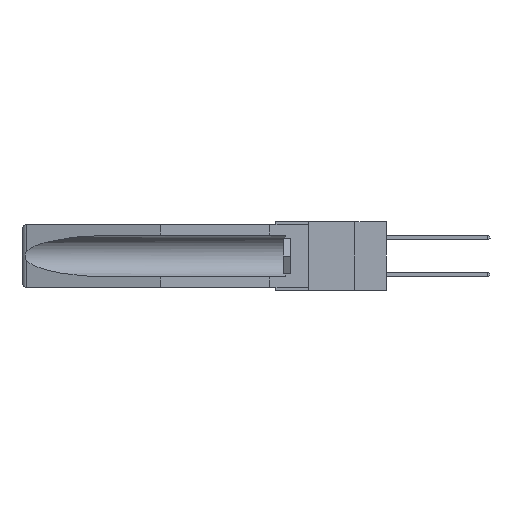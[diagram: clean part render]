
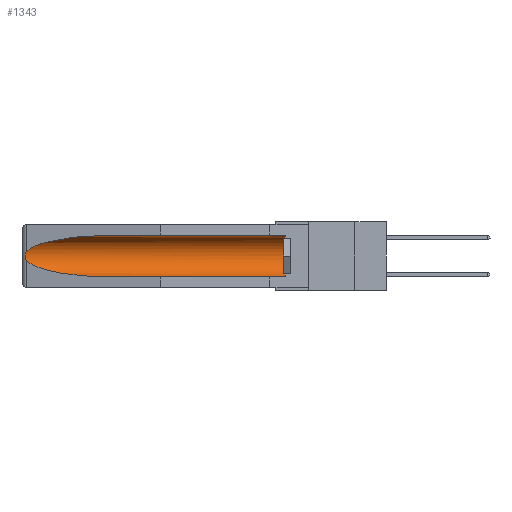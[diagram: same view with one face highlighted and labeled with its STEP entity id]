
A CAD part, left-side view. The second image highlights one B-rep face of the part: STEP entity #1343.
In plain terms, the highlighted cylindrical face has radius 2.857 mm (diameter 5.715 mm), a partial arc.
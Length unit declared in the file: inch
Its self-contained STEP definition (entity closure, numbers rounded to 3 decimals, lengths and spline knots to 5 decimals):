
#374 = CARTESIAN_POINT ( 'NONE',  ( 0.155, -0.30754, -0.284 ) ) ;
#415 = VECTOR ( 'NONE', #24213, 39.37008 ) ;
#1343 = ADVANCED_FACE ( 'NONE', ( #32321 ), #10674, .F. ) ;
#1872 = CARTESIAN_POINT ( 'NONE',  ( 0.155, 0.126, -0.284 ) ) ;
#2726 = EDGE_CURVE ( 'NONE', #32464, #9034, #24548, .T. ) ;
#3020 = CARTESIAN_POINT ( 'NONE',  ( 0.155, -0.30754, -0.1715 ) ) ;
#3129 = DIRECTION ( 'NONE',  ( 0., 1., 0. ) ) ;
#5174 = EDGE_CURVE ( 'NONE', #14724, #9034, #23425, .T. ) ;
#5193 = CARTESIAN_POINT ( 'NONE',  ( 0.155, 1.07973, -0.059 ) ) ;
#5306 = CARTESIAN_POINT ( 'NONE',  ( 0.155, 1.07973, -0.284 ) ) ;
#6300 = VECTOR ( 'NONE', #32778, 39.37008 ) ;
#6371 = DIRECTION ( 'NONE',  ( 0., 0., 1. ) ) ;
#7071 = CARTESIAN_POINT ( 'NONE',  ( 0.155, 0.126, -0.059 ) ) ;
#7737 = CARTESIAN_POINT ( 'NONE',  ( 0.26537, 1.52718, -0.14972 ) ) ;
#7749 = CARTESIAN_POINT ( 'NONE',  ( 0.26537, 1.52718, -0.19328 ) ) ;
#8071 = CARTESIAN_POINT ( 'NONE',  ( 0.26537, 1.52718, -0.19328 ) ) ;
#8982 = VERTEX_POINT ( 'NONE', #10057 ) ;
#9034 = VERTEX_POINT ( 'NONE', #15306 ) ;
#9903 = CARTESIAN_POINT ( 'NONE',  ( 0.26537, 1.52718, -0.14972 ) ) ;
#9992 = EDGE_CURVE ( 'NONE', #14724, #17891, #33779, .T. ) ;
#10057 = CARTESIAN_POINT ( 'NONE',  ( 0.155, 1.07973, -0.059 ) ) ;
#10094 = AXIS2_PLACEMENT_3D ( 'NONE', #16329, #14171, #6371 ) ;
#10490 = CARTESIAN_POINT ( 'NONE',  ( 0.21114, 1.30732, -0.284 ) ) ;
#10674 = CYLINDRICAL_SURFACE ( 'NONE', #21735, 0.1125 ) ;
#10921 = CARTESIAN_POINT ( 'NONE',  ( 0.2675, 1.53308, -0.17534 ) ) ;
#10960 = CARTESIAN_POINT ( 'NONE',  ( 0.26537, 1.52718, -0.19328 ) ) ;
#11031 = CARTESIAN_POINT ( 'NONE',  ( 0.26597, 1.5296, -0.19026 ) ) ;
#12659 = EDGE_CURVE ( 'NONE', #8982, #20902, #20009, .T. ) ;
#12894 = CARTESIAN_POINT ( 'NONE',  ( 0.26537, 1.52718, -0.14972 ) ) ;
#13208 = CARTESIAN_POINT ( 'NONE',  ( 0.26655, 1.53094, -0.18657 ) ) ;
#13767 = ORIENTED_EDGE ( 'NONE', *, *, #12659, .T. ) ;
#14171 = DIRECTION ( 'NONE',  ( 0., -1., 0. ) ) ;
#14724 = VERTEX_POINT ( 'NONE', #1872 ) ;
#14777 = ORIENTED_EDGE ( 'NONE', *, *, #25360, .T. ) ;
#15306 = CARTESIAN_POINT ( 'NONE',  ( 0.155, 1.07973, -0.284 ) ) ;
#15614 = ORIENTED_EDGE ( 'NONE', *, *, #17429, .T. ) ;
#16329 = CARTESIAN_POINT ( 'NONE',  ( 0.155, 0.126, -0.1715 ) ) ;
#17429 = EDGE_CURVE ( 'NONE', #20902, #32464, #27056, .T. ) ;
#17891 = VERTEX_POINT ( 'NONE', #7071 ) ;
#18603 = CARTESIAN_POINT ( 'NONE',  ( 0.2673, 1.5327, -0.16383 ) ) ;
#19686 = CARTESIAN_POINT ( 'NONE',  ( 0.155, -0.30754, -0.059 ) ) ;
#20009 =( BOUNDED_CURVE ( )  B_SPLINE_CURVE ( 3, ( #5193, #20822, #31043, #7737 ),
 .UNSPECIFIED., .F., .F. ) 
 B_SPLINE_CURVE_WITH_KNOTS ( ( 4, 4 ),
 ( 4.71239, 6.08839 ),
 .UNSPECIFIED. ) 
 CURVE ( )  GEOMETRIC_REPRESENTATION_ITEM ( )  RATIONAL_B_SPLINE_CURVE ( ( 1., 0.848, 0.848, 1. ) ) 
 REPRESENTATION_ITEM ( '' )  );
#20822 = CARTESIAN_POINT ( 'NONE',  ( 0.21114, 1.30732, -0.059 ) ) ;
#20902 = VERTEX_POINT ( 'NONE', #9903 ) ;
#21088 = LINE ( 'NONE', #19686, #6300 ) ;
#21462 = CARTESIAN_POINT ( 'NONE',  ( 0.26597, 1.52961, -0.15275 ) ) ;
#21613 = DIRECTION ( 'NONE',  ( 0., 0., 1. ) ) ;
#21694 = ORIENTED_EDGE ( 'NONE', *, *, #9992, .T. ) ;
#21735 = AXIS2_PLACEMENT_3D ( 'NONE', #3020, #3129, #21613 ) ;
#23425 = LINE ( 'NONE', #374, #415 ) ;
#24067 = CARTESIAN_POINT ( 'NONE',  ( 0.2675, 1.53308, -0.16763 ) ) ;
#24213 = DIRECTION ( 'NONE',  ( 0., 1., 0. ) ) ;
#24548 =( BOUNDED_CURVE ( )  B_SPLINE_CURVE ( 3, ( #7749, #31478, #10490, #5306 ),
 .UNSPECIFIED., .F., .F. ) 
 B_SPLINE_CURVE_WITH_KNOTS ( ( 4, 4 ),
 ( 0.1948, 1.5708 ),
 .UNSPECIFIED. ) 
 CURVE ( )  GEOMETRIC_REPRESENTATION_ITEM ( )  RATIONAL_B_SPLINE_CURVE ( ( 1., 0.848, 0.848, 1. ) ) 
 REPRESENTATION_ITEM ( '' )  );
#25360 = EDGE_CURVE ( 'NONE', #17891, #8982, #21088, .T. ) ;
#26691 = CARTESIAN_POINT ( 'NONE',  ( 0.2673, 1.53269, -0.17917 ) ) ;
#27056 = B_SPLINE_CURVE_WITH_KNOTS ( 'NONE', 3,
 ( #12894, #21462, #28895, #18603, #24067, #10921, #26691, #13208, #11031, #8071 ),
 .UNSPECIFIED., .F., .F.,
 ( 4, 2, 2, 2, 4 ),
 ( 0., 0.00029, 0.00058, 0.00087, 0.00117 ),
 .UNSPECIFIED. ) ;
#28845 = EDGE_LOOP ( 'NONE', ( #13767, #15614, #28875, #33050, #21694, #14777 ) ) ;
#28875 = ORIENTED_EDGE ( 'NONE', *, *, #2726, .T. ) ;
#28895 = CARTESIAN_POINT ( 'NONE',  ( 0.26654, 1.53092, -0.15636 ) ) ;
#31043 = CARTESIAN_POINT ( 'NONE',  ( 0.25451, 1.48313, -0.09465 ) ) ;
#31478 = CARTESIAN_POINT ( 'NONE',  ( 0.25451, 1.48313, -0.24835 ) ) ;
#32321 = FACE_OUTER_BOUND ( 'NONE', #28845, .T. ) ;
#32464 = VERTEX_POINT ( 'NONE', #10960 ) ;
#32778 = DIRECTION ( 'NONE',  ( 0., 1., 0. ) ) ;
#33050 = ORIENTED_EDGE ( 'NONE', *, *, #5174, .F. ) ;
#33779 = CIRCLE ( 'NONE', #10094, 0.1125 ) ;
